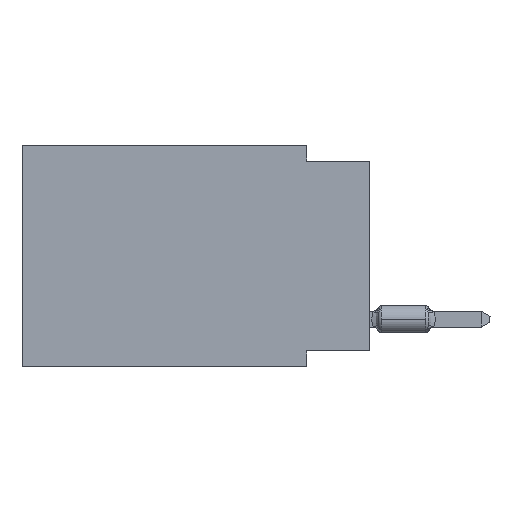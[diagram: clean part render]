
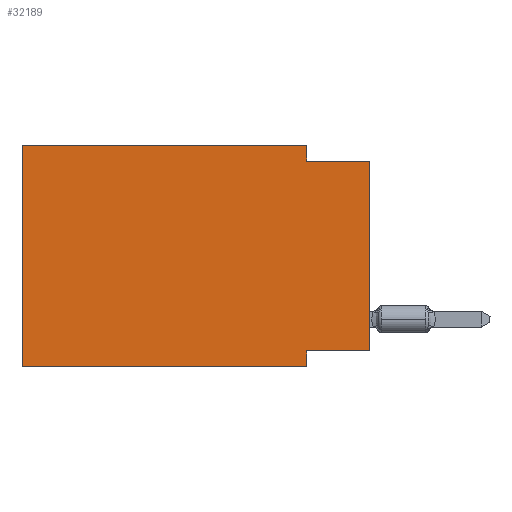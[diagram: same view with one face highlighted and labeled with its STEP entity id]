
A CAD part, left-side view. The second image highlights one B-rep face of the part: STEP entity #32189.
In plain terms, the highlighted planar face has unit normal (-1, 0, 0).
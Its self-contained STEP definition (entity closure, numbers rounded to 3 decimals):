
#1168 = CARTESIAN_POINT ( 'NONE',  ( 0., 0., -0.635 ) ) ;
#1803 = VECTOR ( 'NONE', #29833, 1000. ) ;
#2670 = CARTESIAN_POINT ( 'NONE',  ( 0., 13.97, 0. ) ) ;
#2800 = VECTOR ( 'NONE', #50545, 1000. ) ;
#3557 = AXIS2_PLACEMENT_3D ( 'NONE', #2670, #32791, #6873 ) ;
#3923 = VERTEX_POINT ( 'NONE', #1168 ) ;
#4215 = VECTOR ( 'NONE', #5187, 1000. ) ;
#5187 = DIRECTION ( 'NONE',  ( 0., -1., 0. ) ) ;
#5861 = CARTESIAN_POINT ( 'NONE',  ( 0., 0., -0.635 ) ) ;
#6010 = CARTESIAN_POINT ( 'NONE',  ( 0., 13.97, -8.89 ) ) ;
#6201 = DIRECTION ( 'NONE',  ( 0., 0., -1. ) ) ;
#6780 = ORIENTED_EDGE ( 'NONE', *, *, #43141, .F. ) ;
#6873 = DIRECTION ( 'NONE',  ( 0., 0., -1. ) ) ;
#7881 = VECTOR ( 'NONE', #40208, 1000. ) ;
#8529 = ORIENTED_EDGE ( 'NONE', *, *, #8955, .F. ) ;
#8653 = EDGE_CURVE ( 'NONE', #54239, #29678, #27595, .T. ) ;
#8955 = EDGE_CURVE ( 'NONE', #29678, #3923, #27000, .T. ) ;
#9317 = CARTESIAN_POINT ( 'NONE',  ( 0., 2.54, 0. ) ) ;
#9331 = LINE ( 'NONE', #14385, #17789 ) ;
#9613 = CARTESIAN_POINT ( 'NONE',  ( 0., 0., -8.255 ) ) ;
#11903 = VERTEX_POINT ( 'NONE', #20899 ) ;
#12482 = EDGE_CURVE ( 'NONE', #45734, #36760, #51213, .T. ) ;
#14385 = CARTESIAN_POINT ( 'NONE',  ( 0., 13.97, 0. ) ) ;
#14921 = ORIENTED_EDGE ( 'NONE', *, *, #37788, .F. ) ;
#16090 = EDGE_CURVE ( 'NONE', #16237, #11903, #48265, .T. ) ;
#16237 = VERTEX_POINT ( 'NONE', #6010 ) ;
#16390 = DIRECTION ( 'NONE',  ( 0., 0., -1. ) ) ;
#17587 = CARTESIAN_POINT ( 'NONE',  ( 0., 13.97, -8.89 ) ) ;
#17789 = VECTOR ( 'NONE', #26509, 1000. ) ;
#19300 = LINE ( 'NONE', #50738, #29432 ) ;
#20702 = LINE ( 'NONE', #29134, #2800 ) ;
#20899 = CARTESIAN_POINT ( 'NONE',  ( 0., 2.54, -8.89 ) ) ;
#22111 = LINE ( 'NONE', #30869, #36127 ) ;
#24301 = VERTEX_POINT ( 'NONE', #35019 ) ;
#26509 = DIRECTION ( 'NONE',  ( 0., 0., 1. ) ) ;
#27000 = LINE ( 'NONE', #5861, #7881 ) ;
#27595 = LINE ( 'NONE', #9317, #33063 ) ;
#28213 = ORIENTED_EDGE ( 'NONE', *, *, #12482, .F. ) ;
#29134 = CARTESIAN_POINT ( 'NONE',  ( 0., 13.97, 0. ) ) ;
#29432 = VECTOR ( 'NONE', #16390, 1000. ) ;
#29576 = EDGE_CURVE ( 'NONE', #45734, #3923, #22111, .T. ) ;
#29678 = VERTEX_POINT ( 'NONE', #35900 ) ;
#29833 = DIRECTION ( 'NONE',  ( 0., 1., 0. ) ) ;
#30223 = ORIENTED_EDGE ( 'NONE', *, *, #8653, .F. ) ;
#30869 = CARTESIAN_POINT ( 'NONE',  ( 0., 0., 0. ) ) ;
#32189 = ADVANCED_FACE ( 'NONE', ( #37564 ), #45467, .F. ) ;
#32791 = DIRECTION ( 'NONE',  ( 1., 0., 0. ) ) ;
#33063 = VECTOR ( 'NONE', #6201, 1000. ) ;
#33474 = DIRECTION ( 'NONE',  ( 0., 0., 1. ) ) ;
#34861 = CARTESIAN_POINT ( 'NONE',  ( 0., 0., -8.255 ) ) ;
#35019 = CARTESIAN_POINT ( 'NONE',  ( 0., 13.97, 0. ) ) ;
#35900 = CARTESIAN_POINT ( 'NONE',  ( 0., 2.54, -0.635 ) ) ;
#36127 = VECTOR ( 'NONE', #33474, 1000. ) ;
#36760 = VERTEX_POINT ( 'NONE', #45910 ) ;
#37564 = FACE_OUTER_BOUND ( 'NONE', #42048, .T. ) ;
#37788 = EDGE_CURVE ( 'NONE', #24301, #54239, #20702, .T. ) ;
#40208 = DIRECTION ( 'NONE',  ( 0., -1., 0. ) ) ;
#42011 = ORIENTED_EDGE ( 'NONE', *, *, #29576, .T. ) ;
#42048 = EDGE_LOOP ( 'NONE', ( #42011, #8529, #30223, #14921, #6780, #48786, #55617, #28213 ) ) ;
#42789 = EDGE_CURVE ( 'NONE', #36760, #11903, #19300, .T. ) ;
#43141 = EDGE_CURVE ( 'NONE', #16237, #24301, #9331, .T. ) ;
#45467 = PLANE ( 'NONE',  #3557 ) ;
#45734 = VERTEX_POINT ( 'NONE', #9613 ) ;
#45787 = CARTESIAN_POINT ( 'NONE',  ( 0., 2.54, 0. ) ) ;
#45910 = CARTESIAN_POINT ( 'NONE',  ( 0., 2.54, -8.255 ) ) ;
#48265 = LINE ( 'NONE', #17587, #4215 ) ;
#48786 = ORIENTED_EDGE ( 'NONE', *, *, #16090, .T. ) ;
#50545 = DIRECTION ( 'NONE',  ( 0., -1., 0. ) ) ;
#50738 = CARTESIAN_POINT ( 'NONE',  ( 0., 2.54, -8.89 ) ) ;
#51213 = LINE ( 'NONE', #34861, #1803 ) ;
#54239 = VERTEX_POINT ( 'NONE', #45787 ) ;
#55617 = ORIENTED_EDGE ( 'NONE', *, *, #42789, .F. ) ;
